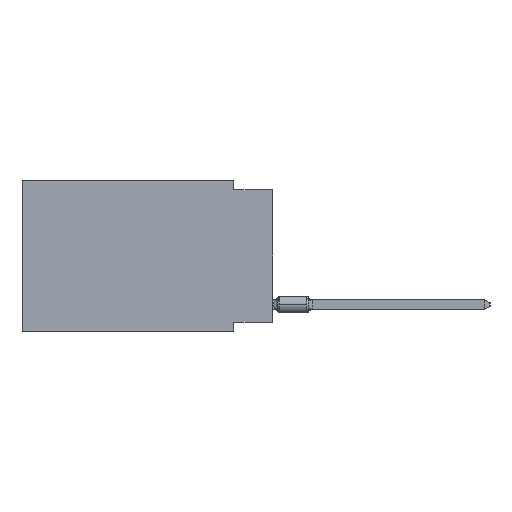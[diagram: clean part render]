
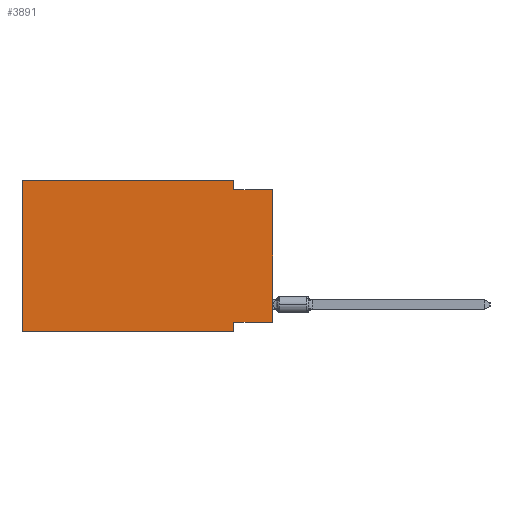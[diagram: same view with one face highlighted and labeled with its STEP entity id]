
A CAD part, left-side view. The second image highlights one B-rep face of the part: STEP entity #3891.
In plain terms, the highlighted planar face has unit normal (-1, 0, 0).
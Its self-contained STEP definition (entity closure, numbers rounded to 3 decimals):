
#1107 = VERTEX_POINT ( 'NONE', #10174 ) ;
#2305 = ORIENTED_EDGE ( 'NONE', *, *, #9394, .F. ) ;
#2577 = LINE ( 'NONE', #11737, #33624 ) ;
#3011 = LINE ( 'NONE', #6474, #25701 ) ;
#3375 = ORIENTED_EDGE ( 'NONE', *, *, #22757, .T. ) ;
#3486 = ORIENTED_EDGE ( 'NONE', *, *, #14261, .F. ) ;
#3769 = ORIENTED_EDGE ( 'NONE', *, *, #18771, .F. ) ;
#3891 = ADVANCED_FACE ( 'NONE', ( #16716 ), #19969, .F. ) ;
#5019 = EDGE_CURVE ( 'NONE', #22407, #20595, #19578, .T. ) ;
#5222 = ORIENTED_EDGE ( 'NONE', *, *, #34583, .F. ) ;
#6474 = CARTESIAN_POINT ( 'NONE',  ( 0., 2.54, -9.906 ) ) ;
#6971 = DIRECTION ( 'NONE',  ( 1., 0., 0. ) ) ;
#7662 = VECTOR ( 'NONE', #8158, 1000. ) ;
#8158 = DIRECTION ( 'NONE',  ( 0., 0., -1. ) ) ;
#8816 = CARTESIAN_POINT ( 'NONE',  ( 0., 16.383, -9.906 ) ) ;
#8936 = CARTESIAN_POINT ( 'NONE',  ( 0., 0., -9.271 ) ) ;
#9394 = EDGE_CURVE ( 'NONE', #22407, #16809, #38330, .T. ) ;
#10174 = CARTESIAN_POINT ( 'NONE',  ( 0., 2.54, -0.635 ) ) ;
#10912 = DIRECTION ( 'NONE',  ( 0., -1., 0. ) ) ;
#11737 = CARTESIAN_POINT ( 'NONE',  ( 0., 0., -9.271 ) ) ;
#12332 = CARTESIAN_POINT ( 'NONE',  ( 0., 2.54, 0. ) ) ;
#13755 = DIRECTION ( 'NONE',  ( 0., 0., 1. ) ) ;
#13885 = DIRECTION ( 'NONE',  ( 0., -1., 0. ) ) ;
#14261 = EDGE_CURVE ( 'NONE', #27598, #20595, #3011, .T. ) ;
#15385 = VECTOR ( 'NONE', #22187, 1000. ) ;
#15879 = LINE ( 'NONE', #21018, #15385 ) ;
#16326 = CARTESIAN_POINT ( 'NONE',  ( 0., 16.383, 0. ) ) ;
#16716 = FACE_OUTER_BOUND ( 'NONE', #17744, .T. ) ;
#16784 = CARTESIAN_POINT ( 'NONE',  ( 0., 0., -0.635 ) ) ;
#16809 = VERTEX_POINT ( 'NONE', #37749 ) ;
#17017 = EDGE_CURVE ( 'NONE', #18464, #27598, #2577, .T. ) ;
#17345 = VECTOR ( 'NONE', #10912, 1000. ) ;
#17744 = EDGE_LOOP ( 'NONE', ( #3375, #5222, #3769, #19971, #2305, #26602, #3486, #33252 ) ) ;
#18464 = VERTEX_POINT ( 'NONE', #8936 ) ;
#18651 = DIRECTION ( 'NONE',  ( 0., 0., -1. ) ) ;
#18771 = EDGE_CURVE ( 'NONE', #27256, #1107, #39042, .T. ) ;
#19360 = DIRECTION ( 'NONE',  ( 0., 0., -1. ) ) ;
#19518 = AXIS2_PLACEMENT_3D ( 'NONE', #16326, #6971, #19360 ) ;
#19578 = LINE ( 'NONE', #32376, #31148 ) ;
#19969 = PLANE ( 'NONE',  #19518 ) ;
#19971 = ORIENTED_EDGE ( 'NONE', *, *, #34710, .F. ) ;
#20595 = VERTEX_POINT ( 'NONE', #26216 ) ;
#21018 = CARTESIAN_POINT ( 'NONE',  ( 0., 16.383, 0. ) ) ;
#22187 = DIRECTION ( 'NONE',  ( 0., -1., 0. ) ) ;
#22374 = CARTESIAN_POINT ( 'NONE',  ( 0., 2.54, -9.271 ) ) ;
#22407 = VERTEX_POINT ( 'NONE', #8816 ) ;
#22757 = EDGE_CURVE ( 'NONE', #18464, #38654, #28799, .T. ) ;
#22889 = CARTESIAN_POINT ( 'NONE',  ( 0., 16.383, 0. ) ) ;
#22998 = CARTESIAN_POINT ( 'NONE',  ( 0., 2.54, 0. ) ) ;
#23900 = DIRECTION ( 'NONE',  ( 0., 1., 0. ) ) ;
#25545 = VECTOR ( 'NONE', #13755, 1000. ) ;
#25701 = VECTOR ( 'NONE', #18651, 1000. ) ;
#26216 = CARTESIAN_POINT ( 'NONE',  ( 0., 2.54, -9.906 ) ) ;
#26602 = ORIENTED_EDGE ( 'NONE', *, *, #5019, .T. ) ;
#27256 = VERTEX_POINT ( 'NONE', #12332 ) ;
#27598 = VERTEX_POINT ( 'NONE', #22374 ) ;
#28799 = LINE ( 'NONE', #38721, #36820 ) ;
#31148 = VECTOR ( 'NONE', #13885, 1000. ) ;
#32069 = CARTESIAN_POINT ( 'NONE',  ( 0., 0., -0.635 ) ) ;
#32376 = CARTESIAN_POINT ( 'NONE',  ( 0., 16.383, -9.906 ) ) ;
#32640 = DIRECTION ( 'NONE',  ( 0., 0., 1. ) ) ;
#33252 = ORIENTED_EDGE ( 'NONE', *, *, #17017, .F. ) ;
#33624 = VECTOR ( 'NONE', #23900, 1000. ) ;
#34583 = EDGE_CURVE ( 'NONE', #1107, #38654, #39124, .T. ) ;
#34710 = EDGE_CURVE ( 'NONE', #16809, #27256, #15879, .T. ) ;
#36820 = VECTOR ( 'NONE', #32640, 1000. ) ;
#37749 = CARTESIAN_POINT ( 'NONE',  ( 0., 16.383, 0. ) ) ;
#38330 = LINE ( 'NONE', #22889, #25545 ) ;
#38654 = VERTEX_POINT ( 'NONE', #32069 ) ;
#38721 = CARTESIAN_POINT ( 'NONE',  ( 0., 0., 0. ) ) ;
#39042 = LINE ( 'NONE', #22998, #7662 ) ;
#39124 = LINE ( 'NONE', #16784, #17345 ) ;
